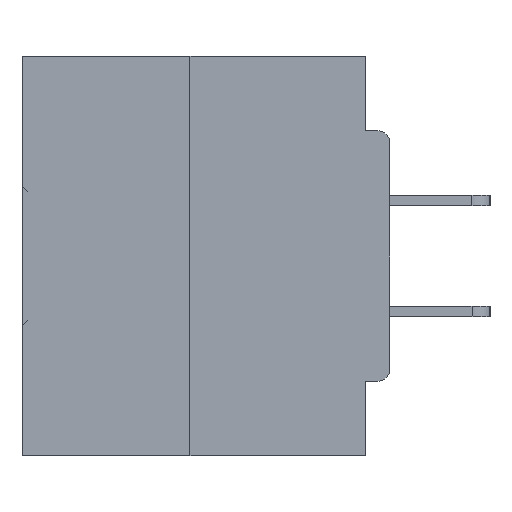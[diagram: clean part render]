
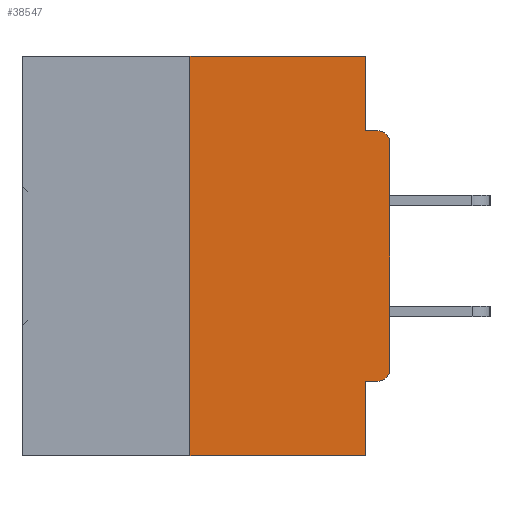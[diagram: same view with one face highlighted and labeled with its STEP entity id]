
A CAD part, left-side view. The second image highlights one B-rep face of the part: STEP entity #38547.
In plain terms, the highlighted planar face has unit normal (-1, 0, 0).
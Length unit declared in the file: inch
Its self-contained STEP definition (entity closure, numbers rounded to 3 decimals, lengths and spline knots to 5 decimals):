
#97 = ORIENTED_EDGE ( 'NONE', *, *, #1616, .F. ) ;
#229 = DIRECTION ( 'NONE',  ( -1., 0., 0. ) ) ;
#1078 = CARTESIAN_POINT ( 'NONE',  ( 0., 0.25, -0.5 ) ) ;
#1616 = EDGE_CURVE ( 'NONE', #35726, #16136, #31033, .T. ) ;
#2508 = LINE ( 'NONE', #37022, #13632 ) ;
#2712 = CARTESIAN_POINT ( 'NONE',  ( 0., 0.015, -0.3915 ) ) ;
#2777 = DIRECTION ( 'NONE',  ( 0., 0., -1. ) ) ;
#3017 = LINE ( 'NONE', #28291, #14741 ) ;
#4566 = CARTESIAN_POINT ( 'NONE',  ( 0., 0., -0.0935 ) ) ;
#4763 = DIRECTION ( 'NONE',  ( 0., 0., -1. ) ) ;
#4813 = ORIENTED_EDGE ( 'NONE', *, *, #6770, .F. ) ;
#4909 = CARTESIAN_POINT ( 'NONE',  ( 0., 0.46, -0.5 ) ) ;
#5033 = VERTEX_POINT ( 'NONE', #12453 ) ;
#5746 = LINE ( 'NONE', #27769, #9094 ) ;
#5870 = AXIS2_PLACEMENT_3D ( 'NONE', #2712, #10178, #45205 ) ;
#6046 = ORIENTED_EDGE ( 'NONE', *, *, #7511, .T. ) ;
#6222 = CARTESIAN_POINT ( 'NONE',  ( 0., 0.25, 0. ) ) ;
#6591 = EDGE_CURVE ( 'NONE', #41154, #28712, #3017, .T. ) ;
#6770 = EDGE_CURVE ( 'NONE', #30640, #35146, #27061, .T. ) ;
#6992 = CARTESIAN_POINT ( 'NONE',  ( 0., 0.031, -0.5 ) ) ;
#7078 = EDGE_CURVE ( 'NONE', #5033, #22700, #5746, .T. ) ;
#7511 = EDGE_CURVE ( 'NONE', #13477, #5033, #24721, .T. ) ;
#7867 = AXIS2_PLACEMENT_3D ( 'NONE', #31263, #41421, #45047 ) ;
#8854 = CARTESIAN_POINT ( 'NONE',  ( 0., 0.015, -0.4065 ) ) ;
#9094 = VECTOR ( 'NONE', #41813, 39.37008 ) ;
#10178 = DIRECTION ( 'NONE',  ( -1., 0., 0. ) ) ;
#10425 = DIRECTION ( 'NONE',  ( 0., -1., 0. ) ) ;
#10872 = LINE ( 'NONE', #4909, #38245 ) ;
#12078 = ORIENTED_EDGE ( 'NONE', *, *, #17965, .F. ) ;
#12453 = CARTESIAN_POINT ( 'NONE',  ( 0., 0., -0.3915 ) ) ;
#13477 = VERTEX_POINT ( 'NONE', #8854 ) ;
#13632 = VECTOR ( 'NONE', #4763, 39.37008 ) ;
#14741 = VECTOR ( 'NONE', #20780, 39.37008 ) ;
#15772 = CARTESIAN_POINT ( 'NONE',  ( 0., 0.031, -0.0935 ) ) ;
#16136 = VERTEX_POINT ( 'NONE', #44072 ) ;
#17965 = EDGE_CURVE ( 'NONE', #13477, #30640, #34906, .T. ) ;
#18053 = CARTESIAN_POINT ( 'NONE',  ( 0., 0.015, -0.1085 ) ) ;
#18919 = DIRECTION ( 'NONE',  ( 0., -1., 0. ) ) ;
#19212 = VECTOR ( 'NONE', #2777, 39.37008 ) ;
#19451 = DIRECTION ( 'NONE',  ( 0., -1., 0. ) ) ;
#20522 = PLANE ( 'NONE',  #7867 ) ;
#20780 = DIRECTION ( 'NONE',  ( 0., 0., 1. ) ) ;
#22700 = VERTEX_POINT ( 'NONE', #45399 ) ;
#23071 = ORIENTED_EDGE ( 'NONE', *, *, #43255, .T. ) ;
#23340 = ORIENTED_EDGE ( 'NONE', *, *, #43315, .F. ) ;
#23838 = CARTESIAN_POINT ( 'NONE',  ( 0., 0.031, 0. ) ) ;
#24193 = ORIENTED_EDGE ( 'NONE', *, *, #6591, .F. ) ;
#24721 = CIRCLE ( 'NONE', #5870, 0.015 ) ;
#25846 = ORIENTED_EDGE ( 'NONE', *, *, #41423, .F. ) ;
#27061 = LINE ( 'NONE', #41678, #19212 ) ;
#27769 = CARTESIAN_POINT ( 'NONE',  ( 0., 0., 0. ) ) ;
#28291 = CARTESIAN_POINT ( 'NONE',  ( 0., 0.25, 0. ) ) ;
#28712 = VERTEX_POINT ( 'NONE', #6222 ) ;
#29176 = DIRECTION ( 'NONE',  ( 0., 0., -1. ) ) ;
#30640 = VERTEX_POINT ( 'NONE', #34482 ) ;
#30907 = CARTESIAN_POINT ( 'NONE',  ( 0., 0.46, 0. ) ) ;
#31033 = LINE ( 'NONE', #4566, #34876 ) ;
#31159 = EDGE_LOOP ( 'NONE', ( #25846, #24193, #23071, #4813, #12078, #6046, #35572, #40697, #97, #23340 ) ) ;
#31263 = CARTESIAN_POINT ( 'NONE',  ( 0., 0.46, 0. ) ) ;
#33895 = VERTEX_POINT ( 'NONE', #23838 ) ;
#34008 = DIRECTION ( 'NONE',  ( 0., 1., 0. ) ) ;
#34119 = EDGE_CURVE ( 'NONE', #22700, #16136, #43189, .T. ) ;
#34482 = CARTESIAN_POINT ( 'NONE',  ( 0., 0.031, -0.4065 ) ) ;
#34876 = VECTOR ( 'NONE', #18919, 39.37008 ) ;
#34906 = LINE ( 'NONE', #44977, #41681 ) ;
#35146 = VERTEX_POINT ( 'NONE', #6992 ) ;
#35572 = ORIENTED_EDGE ( 'NONE', *, *, #7078, .T. ) ;
#35726 = VERTEX_POINT ( 'NONE', #15772 ) ;
#37022 = CARTESIAN_POINT ( 'NONE',  ( 0., 0.031, 0. ) ) ;
#38245 = VECTOR ( 'NONE', #19451, 39.37008 ) ;
#38547 = ADVANCED_FACE ( 'NONE', ( #42302 ), #20522, .F. ) ;
#40697 = ORIENTED_EDGE ( 'NONE', *, *, #34119, .T. ) ;
#41154 = VERTEX_POINT ( 'NONE', #1078 ) ;
#41421 = DIRECTION ( 'NONE',  ( 1., 0., 0. ) ) ;
#41423 = EDGE_CURVE ( 'NONE', #28712, #33895, #44268, .T. ) ;
#41678 = CARTESIAN_POINT ( 'NONE',  ( 0., 0.031, -0.5 ) ) ;
#41681 = VECTOR ( 'NONE', #34008, 39.37008 ) ;
#41813 = DIRECTION ( 'NONE',  ( 0., 0., 1. ) ) ;
#42302 = FACE_OUTER_BOUND ( 'NONE', #31159, .T. ) ;
#43189 = CIRCLE ( 'NONE', #44558, 0.015 ) ;
#43255 = EDGE_CURVE ( 'NONE', #41154, #35146, #10872, .T. ) ;
#43315 = EDGE_CURVE ( 'NONE', #33895, #35726, #2508, .T. ) ;
#43695 = VECTOR ( 'NONE', #10425, 39.37008 ) ;
#44072 = CARTESIAN_POINT ( 'NONE',  ( 0., 0.015, -0.0935 ) ) ;
#44268 = LINE ( 'NONE', #30907, #43695 ) ;
#44558 = AXIS2_PLACEMENT_3D ( 'NONE', #18053, #229, #29176 ) ;
#44977 = CARTESIAN_POINT ( 'NONE',  ( 0., 0., -0.4065 ) ) ;
#45047 = DIRECTION ( 'NONE',  ( 0., 0., -1. ) ) ;
#45205 = DIRECTION ( 'NONE',  ( 0., 0., -1. ) ) ;
#45399 = CARTESIAN_POINT ( 'NONE',  ( 0., 0., -0.1085 ) ) ;
